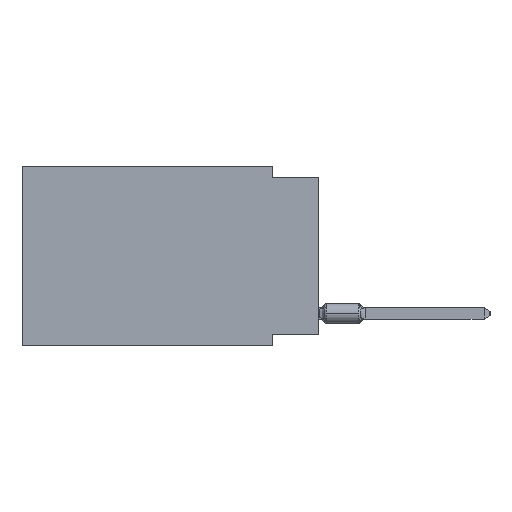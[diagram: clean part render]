
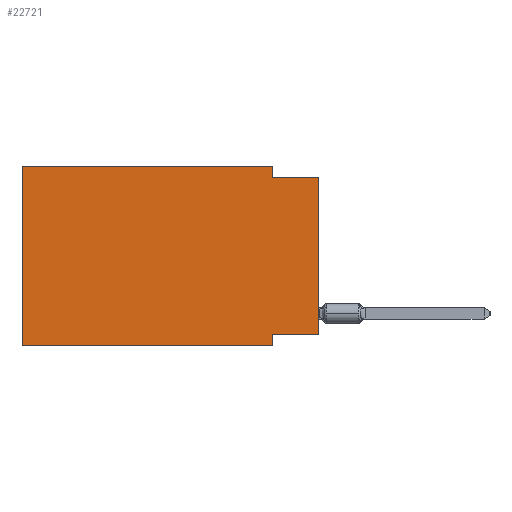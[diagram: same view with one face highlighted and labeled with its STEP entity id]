
A CAD part, left-side view. The second image highlights one B-rep face of the part: STEP entity #22721.
In plain terms, the highlighted planar face has unit normal (-1, 0, 0).
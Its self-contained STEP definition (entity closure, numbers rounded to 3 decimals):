
#199 = CARTESIAN_POINT ( 'NONE',  ( 0., 0., -9.271 ) ) ;
#878 = EDGE_CURVE ( 'NONE', #7357, #35420, #33054, .T. ) ;
#1797 = ORIENTED_EDGE ( 'NONE', *, *, #74095, .F. ) ;
#3729 = DIRECTION ( 'NONE',  ( 0., 0., -1. ) ) ;
#3968 = VECTOR ( 'NONE', #7303, 1000. ) ;
#5959 = ORIENTED_EDGE ( 'NONE', *, *, #44033, .F. ) ;
#6338 = LINE ( 'NONE', #199, #19881 ) ;
#7001 = LINE ( 'NONE', #42227, #63272 ) ;
#7303 = DIRECTION ( 'NONE',  ( 0., 0., 1. ) ) ;
#7357 = VERTEX_POINT ( 'NONE', #39747 ) ;
#7445 = CARTESIAN_POINT ( 'NONE',  ( 0., 2.54, -0.635 ) ) ;
#10021 = DIRECTION ( 'NONE',  ( 1., 0., 0. ) ) ;
#11172 = VERTEX_POINT ( 'NONE', #64144 ) ;
#11321 = DIRECTION ( 'NONE',  ( 0., 1., 0. ) ) ;
#12235 = ORIENTED_EDGE ( 'NONE', *, *, #878, .F. ) ;
#12858 = LINE ( 'NONE', #53096, #15450 ) ;
#13347 = VERTEX_POINT ( 'NONE', #73305 ) ;
#14152 = VECTOR ( 'NONE', #3729, 1000. ) ;
#15450 = VECTOR ( 'NONE', #23600, 1000. ) ;
#15773 = CARTESIAN_POINT ( 'NONE',  ( 0., 16.383, 0. ) ) ;
#16034 = EDGE_CURVE ( 'NONE', #35420, #37971, #12858, .T. ) ;
#16560 = DIRECTION ( 'NONE',  ( 0., -1., 0. ) ) ;
#17231 = VERTEX_POINT ( 'NONE', #43899 ) ;
#18432 = VERTEX_POINT ( 'NONE', #61265 ) ;
#19438 = LINE ( 'NONE', #49324, #14152 ) ;
#19881 = VECTOR ( 'NONE', #11321, 1000. ) ;
#19951 = ORIENTED_EDGE ( 'NONE', *, *, #55295, .F. ) ;
#20782 = EDGE_CURVE ( 'NONE', #11172, #18432, #19438, .T. ) ;
#22419 = DIRECTION ( 'NONE',  ( 0., 0., 1. ) ) ;
#22519 = VECTOR ( 'NONE', #16560, 1000. ) ;
#22721 = ADVANCED_FACE ( 'NONE', ( #23386 ), #46763, .F. ) ;
#23176 = LINE ( 'NONE', #69187, #53944 ) ;
#23386 = FACE_OUTER_BOUND ( 'NONE', #40964, .T. ) ;
#23600 = DIRECTION ( 'NONE',  ( 0., 0., -1. ) ) ;
#24138 = EDGE_CURVE ( 'NONE', #13347, #17231, #30274, .T. ) ;
#25278 = CARTESIAN_POINT ( 'NONE',  ( 0., 0., 0. ) ) ;
#25601 = LINE ( 'NONE', #54730, #39876 ) ;
#30274 = LINE ( 'NONE', #25278, #3968 ) ;
#33054 = LINE ( 'NONE', #44542, #22519 ) ;
#33984 = EDGE_CURVE ( 'NONE', #61516, #18432, #7001, .T. ) ;
#35420 = VERTEX_POINT ( 'NONE', #73734 ) ;
#36735 = DIRECTION ( 'NONE',  ( 0., -1., 0. ) ) ;
#37971 = VERTEX_POINT ( 'NONE', #7445 ) ;
#39747 = CARTESIAN_POINT ( 'NONE',  ( 0., 16.383, 0. ) ) ;
#39876 = VECTOR ( 'NONE', #36735, 1000. ) ;
#40471 = ORIENTED_EDGE ( 'NONE', *, *, #16034, .F. ) ;
#40964 = EDGE_LOOP ( 'NONE', ( #72654, #19951, #40471, #12235, #1797, #53187, #42852, #5959 ) ) ;
#42227 = CARTESIAN_POINT ( 'NONE',  ( 0., 16.383, -9.906 ) ) ;
#42852 = ORIENTED_EDGE ( 'NONE', *, *, #20782, .F. ) ;
#43899 = CARTESIAN_POINT ( 'NONE',  ( 0., 0., -0.635 ) ) ;
#44033 = EDGE_CURVE ( 'NONE', #13347, #11172, #6338, .T. ) ;
#44542 = CARTESIAN_POINT ( 'NONE',  ( 0., 16.383, 0. ) ) ;
#46763 = PLANE ( 'NONE',  #63734 ) ;
#49324 = CARTESIAN_POINT ( 'NONE',  ( 0., 2.54, -9.906 ) ) ;
#51001 = DIRECTION ( 'NONE',  ( 0., 0., -1. ) ) ;
#53096 = CARTESIAN_POINT ( 'NONE',  ( 0., 2.54, 0. ) ) ;
#53187 = ORIENTED_EDGE ( 'NONE', *, *, #33984, .T. ) ;
#53944 = VECTOR ( 'NONE', #22419, 1000. ) ;
#54730 = CARTESIAN_POINT ( 'NONE',  ( 0., 0., -0.635 ) ) ;
#54756 = CARTESIAN_POINT ( 'NONE',  ( 0., 16.383, -9.906 ) ) ;
#55295 = EDGE_CURVE ( 'NONE', #37971, #17231, #25601, .T. ) ;
#59876 = DIRECTION ( 'NONE',  ( 0., -1., 0. ) ) ;
#61265 = CARTESIAN_POINT ( 'NONE',  ( 0., 2.54, -9.906 ) ) ;
#61516 = VERTEX_POINT ( 'NONE', #54756 ) ;
#63272 = VECTOR ( 'NONE', #59876, 1000. ) ;
#63734 = AXIS2_PLACEMENT_3D ( 'NONE', #15773, #10021, #51001 ) ;
#64144 = CARTESIAN_POINT ( 'NONE',  ( 0., 2.54, -9.271 ) ) ;
#69187 = CARTESIAN_POINT ( 'NONE',  ( 0., 16.383, 0. ) ) ;
#72654 = ORIENTED_EDGE ( 'NONE', *, *, #24138, .T. ) ;
#73305 = CARTESIAN_POINT ( 'NONE',  ( 0., 0., -9.271 ) ) ;
#73734 = CARTESIAN_POINT ( 'NONE',  ( 0., 2.54, 0. ) ) ;
#74095 = EDGE_CURVE ( 'NONE', #61516, #7357, #23176, .T. ) ;
